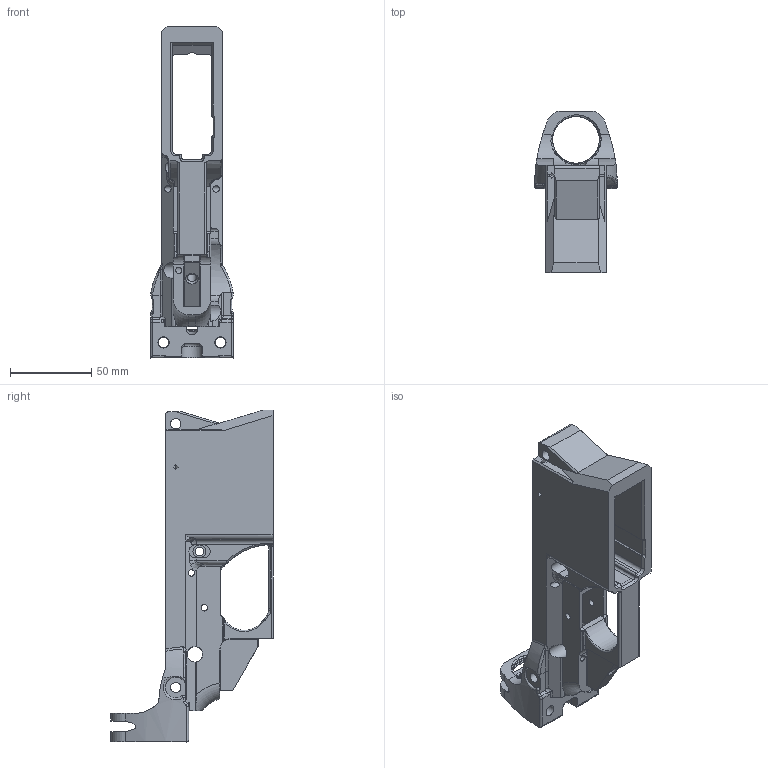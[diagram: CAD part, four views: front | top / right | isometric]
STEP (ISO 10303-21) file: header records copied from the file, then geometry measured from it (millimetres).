
FILE_DESCRIPTION(/* description */ (''),/* implementation_level */ '2;1');
FILE_NAME(/* name */ 'U-Bolt Vanguard.stp',/* time_stamp */ '2020-05-26T12:09:19-05:00',/* author */ ('johne'),/* organization */ (''),/* preprocessor_version */ 'ST-DEVELOPER v18',/* originating_system */ 'Autodesk Inventor 2020',/* authorisation */ '');
FILE_SCHEMA (('AUTOMOTIVE_DESIGN { 1 0 10303 214 3 1 1 }'));
Length unit declared in the file: inch
Products named in the file (1): Vanguard - Fixed Dimensions V1.10
Bounding box: 50.81 x 99.44 x 203.77 mm (x, y, z)
Volume: 184382.2 mm3; surface area: 65571.2 mm2
Topology: 1 solids, 1 shells, 565 faces, 1684 edges, 1092 vertices
Faces by surface type: cylinder 222, plane 174, bspline 114, torus 30, cone 19, sphere 6
Full cylindrical faces by diameter (mm): 3.81 x1, 3.969 x5, 5.182 x1, 5.334 x1, 6.35 x4, 6.477 x1, 6.858 x3, 7.938 x1, 9.55 x2, 28.651 x8
Entity records: 28454 total; most frequent: CARTESIAN_POINT 14212, ORIENTED_EDGE 3340, DIRECTION 2520, EDGE_CURVE 1670, VERTEX_POINT 1092, AXIS2_PLACEMENT_3D 905, LINE 710, VECTOR 710
